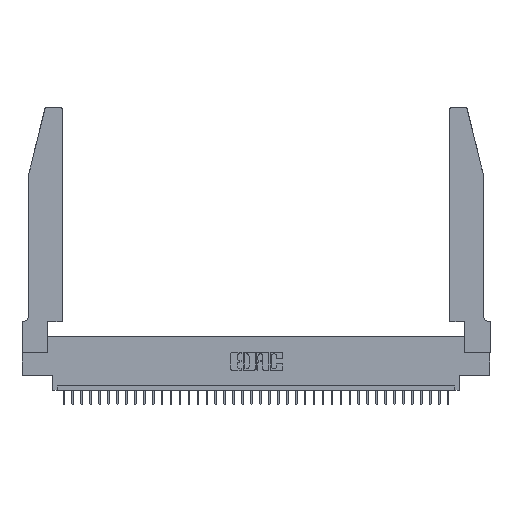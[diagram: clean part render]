
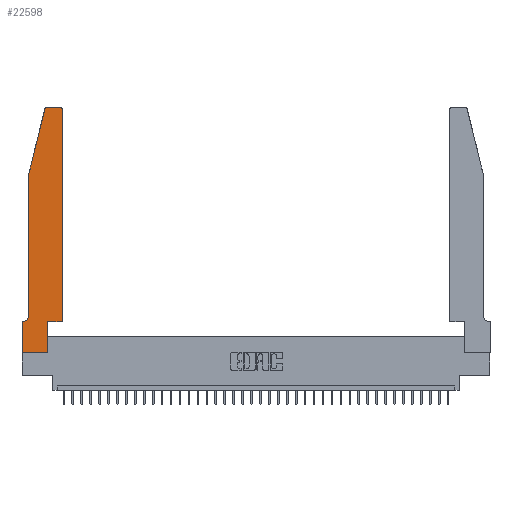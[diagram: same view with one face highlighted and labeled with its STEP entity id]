
A CAD part, top view. The second image highlights one B-rep face of the part: STEP entity #22598.
In plain terms, the highlighted planar face has unit normal (0, 0, 1).
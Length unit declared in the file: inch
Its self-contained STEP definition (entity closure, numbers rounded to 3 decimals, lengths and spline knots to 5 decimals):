
#20 = LINE ( 'NONE', #32903, #30222 ) ;
#400 = ORIENTED_EDGE ( 'NONE', *, *, #21714, .T. ) ;
#692 = DIRECTION ( 'NONE',  ( -0.239, -0.971, 0. ) ) ;
#760 = DIRECTION ( 'NONE',  ( 1., 0., 0. ) ) ;
#1206 = ORIENTED_EDGE ( 'NONE', *, *, #34455, .T. ) ;
#2041 = EDGE_CURVE ( 'NONE', #6579, #25253, #9031, .T. ) ;
#2301 = ORIENTED_EDGE ( 'NONE', *, *, #18678, .T. ) ;
#3040 = LINE ( 'NONE', #7694, #3455 ) ;
#3381 = ORIENTED_EDGE ( 'NONE', *, *, #13460, .T. ) ;
#3386 = VECTOR ( 'NONE', #3554, 39.37008 ) ;
#3442 = LINE ( 'NONE', #37290, #22279 ) ;
#3455 = VECTOR ( 'NONE', #10592, 39.37008 ) ;
#3554 = DIRECTION ( 'NONE',  ( 0., -1., 0. ) ) ;
#4021 = LINE ( 'NONE', #32655, #13694 ) ;
#4047 = EDGE_CURVE ( 'NONE', #18845, #6579, #19399, .T. ) ;
#4557 = ORIENTED_EDGE ( 'NONE', *, *, #21904, .T. ) ;
#4716 = CARTESIAN_POINT ( 'NONE',  ( 0.284, 2.75, 0.37 ) ) ;
#5186 = EDGE_LOOP ( 'NONE', ( #15230, #8588, #4557, #2301, #400, #31827, #21113, #21757, #15267, #10296, #1206, #3381 ) ) ;
#5415 = VERTEX_POINT ( 'NONE', #6109 ) ;
#5464 = CARTESIAN_POINT ( 'NONE',  ( 0.2865, 0.35, 0.37 ) ) ;
#6109 = CARTESIAN_POINT ( 'NONE',  ( 0.0055, 0.35, 0.37 ) ) ;
#6224 = CARTESIAN_POINT ( 'NONE',  ( 0., 0., 0.37 ) ) ;
#6543 = CARTESIAN_POINT ( 'NONE',  ( 0., 0.35, 0.37 ) ) ;
#6570 = VECTOR ( 'NONE', #22730, 39.37008 ) ;
#6579 = VERTEX_POINT ( 'NONE', #4716 ) ;
#7694 = CARTESIAN_POINT ( 'NONE',  ( 0.4505, 0.35, 0.37 ) ) ;
#8588 = ORIENTED_EDGE ( 'NONE', *, *, #2041, .T. ) ;
#8800 = CARTESIAN_POINT ( 'NONE',  ( 0.25487, 2.72718, 0.37 ) ) ;
#9031 = CIRCLE ( 'NONE', #16282, 0.03 ) ;
#9326 = PLANE ( 'NONE',  #10659 ) ;
#9683 = FACE_OUTER_BOUND ( 'NONE', #5186, .T. ) ;
#9695 = CARTESIAN_POINT ( 'NONE',  ( 0.4505, 2.72, 0.37 ) ) ;
#9891 = CARTESIAN_POINT ( 'NONE',  ( 0., 0.35, 0.37 ) ) ;
#9959 = VERTEX_POINT ( 'NONE', #24765 ) ;
#10084 = CARTESIAN_POINT ( 'NONE',  ( 0.0755, 2., 0.37 ) ) ;
#10296 = ORIENTED_EDGE ( 'NONE', *, *, #16988, .T. ) ;
#10313 = DIRECTION ( 'NONE',  ( 0., 0., 1. ) ) ;
#10439 = VERTEX_POINT ( 'NONE', #9695 ) ;
#10592 = DIRECTION ( 'NONE',  ( 1., 0., 0. ) ) ;
#10659 = AXIS2_PLACEMENT_3D ( 'NONE', #6543, #29812, #760 ) ;
#10734 = LINE ( 'NONE', #23423, #22235 ) ;
#10865 = CARTESIAN_POINT ( 'NONE',  ( 0.2865, 0.35, 0.37 ) ) ;
#11240 = AXIS2_PLACEMENT_3D ( 'NONE', #27754, #10313, #31070 ) ;
#12028 = LINE ( 'NONE', #29883, #34891 ) ;
#12358 = DIRECTION ( 'NONE',  ( 1., 0., 0. ) ) ;
#13460 = EDGE_CURVE ( 'NONE', #10439, #18845, #31014, .T. ) ;
#13637 = AXIS2_PLACEMENT_3D ( 'NONE', #17056, #16935, #29307 ) ;
#13694 = VECTOR ( 'NONE', #29976, 39.37008 ) ;
#14355 = EDGE_CURVE ( 'NONE', #5415, #24297, #20, .T. ) ;
#14511 = VERTEX_POINT ( 'NONE', #10865 ) ;
#15230 = ORIENTED_EDGE ( 'NONE', *, *, #4047, .T. ) ;
#15267 = ORIENTED_EDGE ( 'NONE', *, *, #25783, .T. ) ;
#15455 = VECTOR ( 'NONE', #25911, 39.37008 ) ;
#16282 = AXIS2_PLACEMENT_3D ( 'NONE', #17090, #26030, #12358 ) ;
#16935 = DIRECTION ( 'NONE',  ( 0., 0., -1. ) ) ;
#16988 = EDGE_CURVE ( 'NONE', #14511, #9959, #3040, .T. ) ;
#17056 = CARTESIAN_POINT ( 'NONE',  ( 0.0055, 0.42, 0.37 ) ) ;
#17090 = CARTESIAN_POINT ( 'NONE',  ( 0.284, 2.72, 0.37 ) ) ;
#18678 = EDGE_CURVE ( 'NONE', #24712, #19214, #29950, .T. ) ;
#18845 = VERTEX_POINT ( 'NONE', #24011 ) ;
#19214 = VERTEX_POINT ( 'NONE', #34188 ) ;
#19399 = LINE ( 'NONE', #31252, #6570 ) ;
#21113 = ORIENTED_EDGE ( 'NONE', *, *, #37758, .T. ) ;
#21714 = EDGE_CURVE ( 'NONE', #19214, #5415, #24449, .T. ) ;
#21757 = ORIENTED_EDGE ( 'NONE', *, *, #26685, .T. ) ;
#21904 = EDGE_CURVE ( 'NONE', #25253, #24712, #12028, .T. ) ;
#22235 = VECTOR ( 'NONE', #23648, 39.37008 ) ;
#22279 = VECTOR ( 'NONE', #25992, 39.37008 ) ;
#22598 = ADVANCED_FACE ( 'NONE', ( #9683 ), #9326, .T. ) ;
#22730 = DIRECTION ( 'NONE',  ( -1., 0., 0. ) ) ;
#23423 = CARTESIAN_POINT ( 'NONE',  ( 0.4505, 0.35, 0.37 ) ) ;
#23648 = DIRECTION ( 'NONE',  ( 0., 1., 0. ) ) ;
#24011 = CARTESIAN_POINT ( 'NONE',  ( 0.4205, 2.75, 0.37 ) ) ;
#24297 = VERTEX_POINT ( 'NONE', #9891 ) ;
#24449 = CIRCLE ( 'NONE', #13637, 0.07 ) ;
#24712 = VERTEX_POINT ( 'NONE', #26507 ) ;
#24765 = CARTESIAN_POINT ( 'NONE',  ( 0.4505, 0.35, 0.37 ) ) ;
#25253 = VERTEX_POINT ( 'NONE', #8800 ) ;
#25783 = EDGE_CURVE ( 'NONE', #34875, #14511, #26390, .T. ) ;
#25911 = DIRECTION ( 'NONE',  ( 0., 1., 0. ) ) ;
#25992 = DIRECTION ( 'NONE',  ( 1., 0., 0. ) ) ;
#26030 = DIRECTION ( 'NONE',  ( 0., 0., 1. ) ) ;
#26390 = LINE ( 'NONE', #5464, #15455 ) ;
#26507 = CARTESIAN_POINT ( 'NONE',  ( 0.0755, 2., 0.37 ) ) ;
#26685 = EDGE_CURVE ( 'NONE', #35007, #34875, #3442, .T. ) ;
#27754 = CARTESIAN_POINT ( 'NONE',  ( 0.4205, 2.72, 0.37 ) ) ;
#29307 = DIRECTION ( 'NONE',  ( -1., 0., 0. ) ) ;
#29812 = DIRECTION ( 'NONE',  ( 0., 0., 1. ) ) ;
#29883 = CARTESIAN_POINT ( 'NONE',  ( 0.0755, 2., 0.37 ) ) ;
#29950 = LINE ( 'NONE', #10084, #3386 ) ;
#29976 = DIRECTION ( 'NONE',  ( 0., -1., 0. ) ) ;
#30222 = VECTOR ( 'NONE', #33037, 39.37008 ) ;
#31014 = CIRCLE ( 'NONE', #11240, 0.03 ) ;
#31070 = DIRECTION ( 'NONE',  ( 1., 0., 0. ) ) ;
#31252 = CARTESIAN_POINT ( 'NONE',  ( 0.2605, 2.75, 0.37 ) ) ;
#31827 = ORIENTED_EDGE ( 'NONE', *, *, #14355, .T. ) ;
#32655 = CARTESIAN_POINT ( 'NONE',  ( 0., 0., 0.37 ) ) ;
#32903 = CARTESIAN_POINT ( 'NONE',  ( 0.0755, 0.35, 0.37 ) ) ;
#33037 = DIRECTION ( 'NONE',  ( -1., 0., 0. ) ) ;
#34188 = CARTESIAN_POINT ( 'NONE',  ( 0.0755, 0.42, 0.37 ) ) ;
#34455 = EDGE_CURVE ( 'NONE', #9959, #10439, #10734, .T. ) ;
#34875 = VERTEX_POINT ( 'NONE', #37726 ) ;
#34891 = VECTOR ( 'NONE', #692, 39.37008 ) ;
#35007 = VERTEX_POINT ( 'NONE', #6224 ) ;
#37290 = CARTESIAN_POINT ( 'NONE',  ( 0., 0., 0.37 ) ) ;
#37726 = CARTESIAN_POINT ( 'NONE',  ( 0.2865, 0., 0.37 ) ) ;
#37758 = EDGE_CURVE ( 'NONE', #24297, #35007, #4021, .T. ) ;
